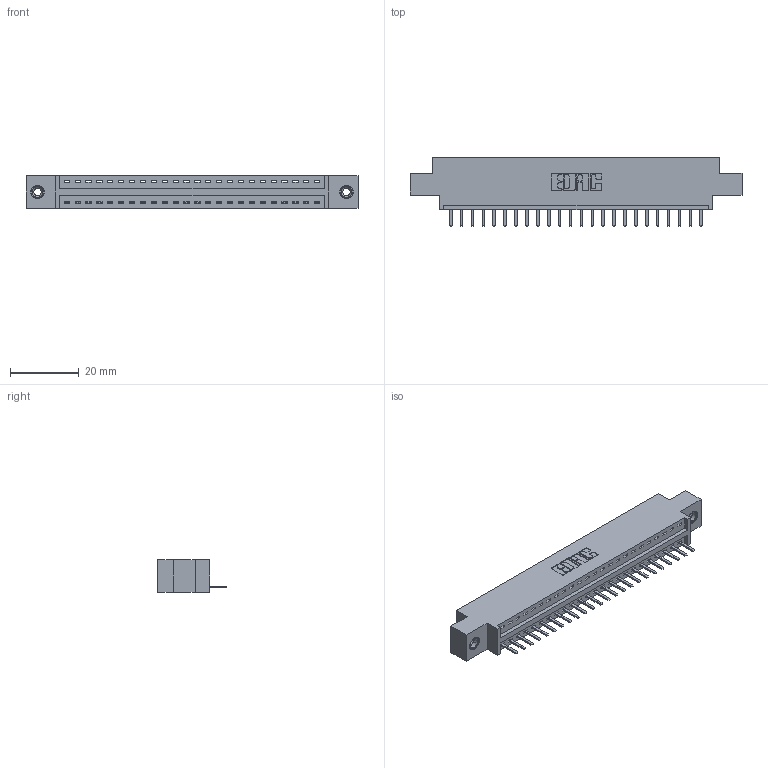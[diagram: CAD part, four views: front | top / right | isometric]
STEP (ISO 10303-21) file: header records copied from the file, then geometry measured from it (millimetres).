
FILE_DESCRIPTION (( 'STEP AP203' ), '1' );
FILE_NAME ('396-024-520-608.STEP', '2018-09-01T12:46:26', ( '' ), ( '' ), 'SwSTEP 2.0', 'SolidWorks 2016', '' );
FILE_SCHEMA (( 'CONFIG_CONTROL_DESIGN' ));
Length unit declared in the file: inch
Products named in the file (4): 346 Part_0.170 Offset - 0.156 Dia-TI; 345-292-001_345-293-120; 345-250-001_345-250-003-102; 396-024-520-608
Assembly tree (27 placements, depth 2):
  396-024-520-608
    346 Part_0.170 Offset - 0.156 Dia-TI
    345-292-001_345-293-120  x24
    345-250-001_345-250-003-102  x2
Bounding box: 96.77 x 20.02 x 9.4 mm (x, y, z)
Volume: 8909.2 mm3; surface area: 10892.8 mm2
Topology: 27 solids, 27 shells, 1674 faces, 4893 edges, 3190 vertices
Faces by surface type: plane 1120, cylinder 538, cone 12, torus 4
Entity records: 18750 total; most frequent: CARTESIAN_POINT 3215, ORIENTED_EDGE 3154, DIRECTION 2871, EDGE_CURVE 1577, VECTOR 1325, LINE 1325, VERTEX_POINT 1044, AXIS2_PLACEMENT_3D 773
